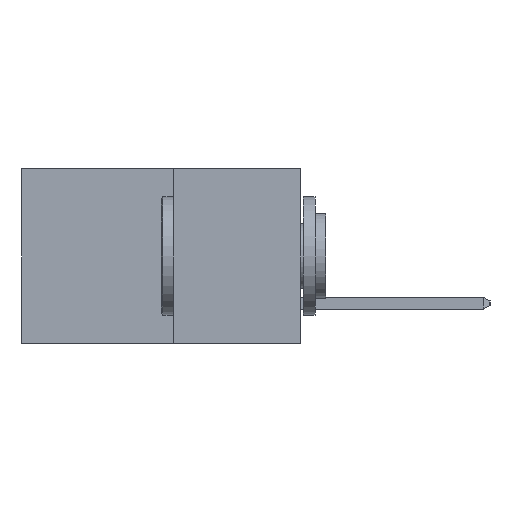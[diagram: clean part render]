
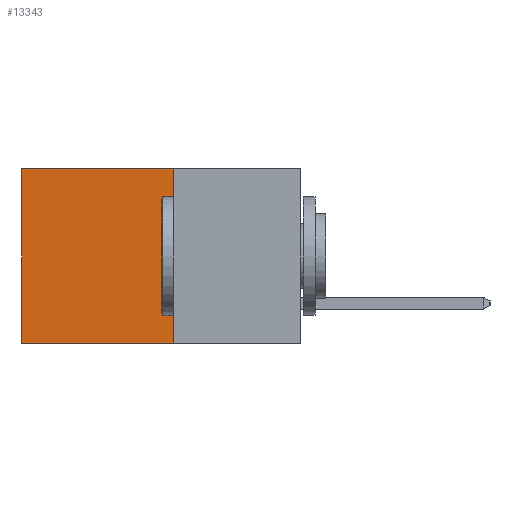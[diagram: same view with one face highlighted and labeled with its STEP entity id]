
A CAD part, left-side view. The second image highlights one B-rep face of the part: STEP entity #13343.
In plain terms, the highlighted planar face has unit normal (-1, 0, 0).
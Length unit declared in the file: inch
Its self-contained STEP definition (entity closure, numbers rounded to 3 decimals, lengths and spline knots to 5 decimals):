
#177 = CARTESIAN_POINT ( 'NONE',  ( 0.277, 0.27, -0.37 ) ) ;
#178 = EDGE_CURVE ( 'NONE', #3242, #6051, #12363, .T. ) ;
#352 = FACE_OUTER_BOUND ( 'NONE', #8881, .T. ) ;
#354 = DIRECTION ( 'NONE',  ( 0., 1., 0. ) ) ;
#473 = CARTESIAN_POINT ( 'NONE',  ( 0.277, 0.27, -0.37 ) ) ;
#1029 = VECTOR ( 'NONE', #6934, 39.37008 ) ;
#1460 = VECTOR ( 'NONE', #13282, 39.37008 ) ;
#1553 = PLANE ( 'NONE',  #2722 ) ;
#1607 = DIRECTION ( 'NONE',  ( 0., 0., -1. ) ) ;
#1938 = CARTESIAN_POINT ( 'NONE',  ( 0.277, 0.59, -0.37 ) ) ;
#2722 = AXIS2_PLACEMENT_3D ( 'NONE', #473, #8001, #1607 ) ;
#2771 = ORIENTED_EDGE ( 'NONE', *, *, #3670, .F. ) ;
#2847 = EDGE_CURVE ( 'NONE', #10189, #7699, #3625, .T. ) ;
#3242 = VERTEX_POINT ( 'NONE', #7518 ) ;
#3388 = DIRECTION ( 'NONE',  ( 0., 0., -1. ) ) ;
#3625 = LINE ( 'NONE', #1938, #11674 ) ;
#3670 = EDGE_CURVE ( 'NONE', #6051, #7699, #6758, .T. ) ;
#3826 = EDGE_CURVE ( 'NONE', #3242, #10189, #8250, .T. ) ;
#5639 = CARTESIAN_POINT ( 'NONE',  ( 0.277, 0.27, -0.37 ) ) ;
#6051 = VERTEX_POINT ( 'NONE', #5639 ) ;
#6758 = LINE ( 'NONE', #177, #1029 ) ;
#6934 = DIRECTION ( 'NONE',  ( 0., 1., 0. ) ) ;
#7518 = CARTESIAN_POINT ( 'NONE',  ( 0.277, 0.27, 0. ) ) ;
#7699 = VERTEX_POINT ( 'NONE', #8668 ) ;
#7922 = VECTOR ( 'NONE', #354, 39.37008 ) ;
#8001 = DIRECTION ( 'NONE',  ( 1., 0., 0. ) ) ;
#8250 = LINE ( 'NONE', #10852, #7922 ) ;
#8668 = CARTESIAN_POINT ( 'NONE',  ( 0.277, 0.59, -0.37 ) ) ;
#8881 = EDGE_LOOP ( 'NONE', ( #12617, #2771, #9101, #9762 ) ) ;
#9101 = ORIENTED_EDGE ( 'NONE', *, *, #178, .F. ) ;
#9762 = ORIENTED_EDGE ( 'NONE', *, *, #3826, .T. ) ;
#10189 = VERTEX_POINT ( 'NONE', #11600 ) ;
#10852 = CARTESIAN_POINT ( 'NONE',  ( 0.277, 0.27, 0. ) ) ;
#11600 = CARTESIAN_POINT ( 'NONE',  ( 0.277, 0.59, 0. ) ) ;
#11674 = VECTOR ( 'NONE', #3388, 39.37008 ) ;
#12363 = LINE ( 'NONE', #13298, #1460 ) ;
#12617 = ORIENTED_EDGE ( 'NONE', *, *, #2847, .T. ) ;
#13282 = DIRECTION ( 'NONE',  ( 0., 0., -1. ) ) ;
#13298 = CARTESIAN_POINT ( 'NONE',  ( 0.277, 0.27, -0.37 ) ) ;
#13343 = ADVANCED_FACE ( 'NONE', ( #352 ), #1553, .F. ) ;
